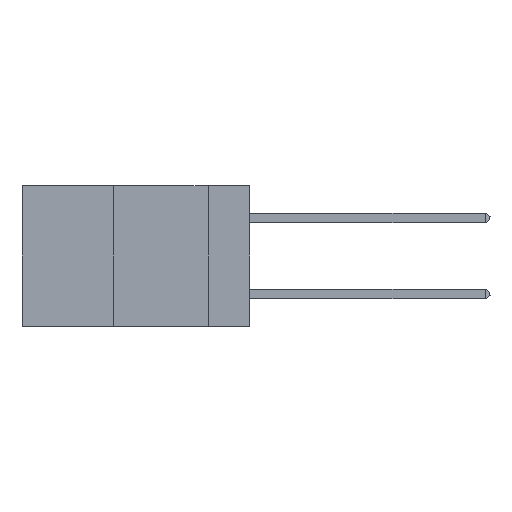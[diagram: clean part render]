
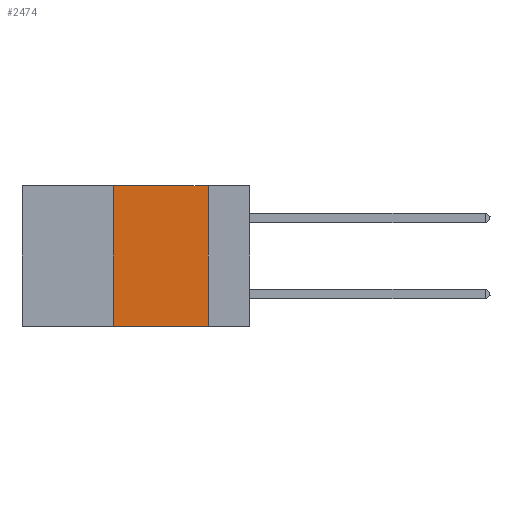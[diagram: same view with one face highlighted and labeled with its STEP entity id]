
A CAD part, left-side view. The second image highlights one B-rep face of the part: STEP entity #2474.
In plain terms, the highlighted planar face has unit normal (-1, 0, 0).
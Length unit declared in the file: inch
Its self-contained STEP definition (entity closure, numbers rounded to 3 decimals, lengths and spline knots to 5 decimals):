
#1250 = DIRECTION ( 'NONE',  ( 0., -1., 0. ) ) ;
#2474 = ADVANCED_FACE ( 'NONE', ( #13944 ), #19692, .F. ) ;
#3926 = VERTEX_POINT ( 'NONE', #24844 ) ;
#4829 = CARTESIAN_POINT ( 'NONE',  ( 0., 0.11, 0. ) ) ;
#7055 = CARTESIAN_POINT ( 'NONE',  ( 0., 0.36, 0. ) ) ;
#9992 = DIRECTION ( 'NONE',  ( 0., -1., 0. ) ) ;
#11658 = EDGE_LOOP ( 'NONE', ( #25911, #21395, #29602, #21615 ) ) ;
#12220 = DIRECTION ( 'NONE',  ( 0., 0., 1. ) ) ;
#12572 = VECTOR ( 'NONE', #1250, 39.37008 ) ;
#13944 = FACE_OUTER_BOUND ( 'NONE', #11658, .T. ) ;
#14348 = VECTOR ( 'NONE', #12220, 39.37008 ) ;
#14408 = VERTEX_POINT ( 'NONE', #16532 ) ;
#16532 = CARTESIAN_POINT ( 'NONE',  ( 0., 0.36, -0.37 ) ) ;
#17898 = CARTESIAN_POINT ( 'NONE',  ( 0., 0.6, 0. ) ) ;
#19110 = AXIS2_PLACEMENT_3D ( 'NONE', #20045, #34089, #25566 ) ;
#19692 = PLANE ( 'NONE',  #19110 ) ;
#20045 = CARTESIAN_POINT ( 'NONE',  ( 0., 0.6, 0. ) ) ;
#20522 = EDGE_CURVE ( 'NONE', #14408, #3926, #22886, .T. ) ;
#20712 = DIRECTION ( 'NONE',  ( 0., 0., -1. ) ) ;
#20821 = VERTEX_POINT ( 'NONE', #27321 ) ;
#21395 = ORIENTED_EDGE ( 'NONE', *, *, #21817, .F. ) ;
#21615 = ORIENTED_EDGE ( 'NONE', *, *, #23395, .T. ) ;
#21817 = EDGE_CURVE ( 'NONE', #3926, #33932, #31568, .T. ) ;
#22751 = CARTESIAN_POINT ( 'NONE',  ( 0., 0.6, -0.37 ) ) ;
#22886 = LINE ( 'NONE', #7055, #14348 ) ;
#23203 = CARTESIAN_POINT ( 'NONE',  ( 0., 0.11, 0. ) ) ;
#23395 = EDGE_CURVE ( 'NONE', #14408, #20821, #34041, .T. ) ;
#24642 = EDGE_CURVE ( 'NONE', #33932, #20821, #34806, .T. ) ;
#24844 = CARTESIAN_POINT ( 'NONE',  ( 0., 0.36, 0. ) ) ;
#25566 = DIRECTION ( 'NONE',  ( 0., 0., -1. ) ) ;
#25911 = ORIENTED_EDGE ( 'NONE', *, *, #24642, .F. ) ;
#26640 = VECTOR ( 'NONE', #20712, 39.37008 ) ;
#27321 = CARTESIAN_POINT ( 'NONE',  ( 0., 0.11, -0.37 ) ) ;
#29602 = ORIENTED_EDGE ( 'NONE', *, *, #20522, .F. ) ;
#30696 = VECTOR ( 'NONE', #9992, 39.37008 ) ;
#31568 = LINE ( 'NONE', #17898, #30696 ) ;
#33932 = VERTEX_POINT ( 'NONE', #4829 ) ;
#34041 = LINE ( 'NONE', #22751, #12572 ) ;
#34089 = DIRECTION ( 'NONE',  ( 1., 0., 0. ) ) ;
#34806 = LINE ( 'NONE', #23203, #26640 ) ;
